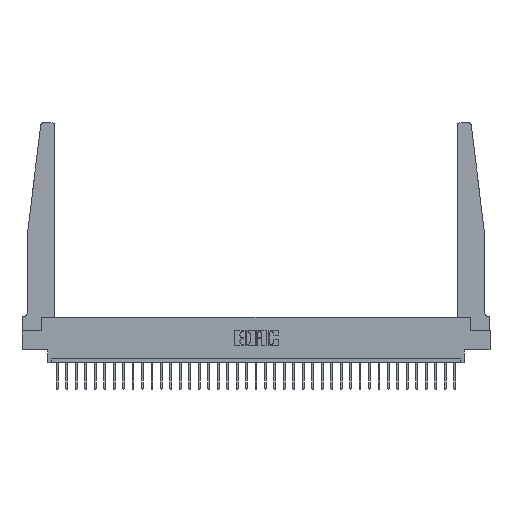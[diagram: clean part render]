
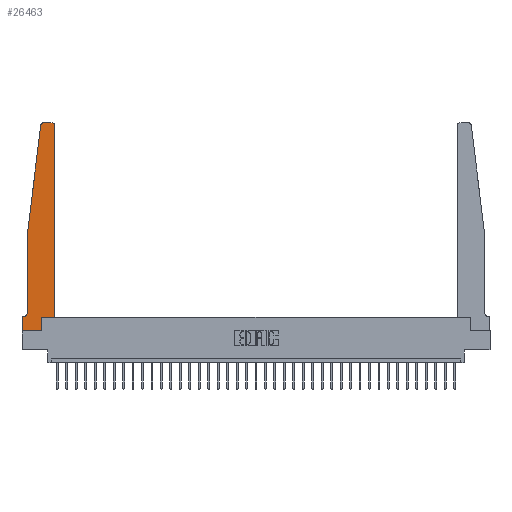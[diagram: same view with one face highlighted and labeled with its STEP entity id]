
A CAD part, top view. The second image highlights one B-rep face of the part: STEP entity #26463.
In plain terms, the highlighted planar face has unit normal (0, 0, 1).
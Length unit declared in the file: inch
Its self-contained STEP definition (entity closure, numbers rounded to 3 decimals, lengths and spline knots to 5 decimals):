
#137 = VERTEX_POINT ( 'NONE', #4157 ) ;
#386 = CARTESIAN_POINT ( 'NONE',  ( 0.27653, 2.72, 0.37 ) ) ;
#509 = VERTEX_POINT ( 'NONE', #14719 ) ;
#3121 = CARTESIAN_POINT ( 'NONE',  ( 0., 0., 0.37 ) ) ;
#3196 = DIRECTION ( 'NONE',  ( 0., -1., 0. ) ) ;
#3237 = LINE ( 'NONE', #26869, #28651 ) ;
#3584 = CARTESIAN_POINT ( 'NONE',  ( 0.425, 2.72, 0.37 ) ) ;
#4157 = CARTESIAN_POINT ( 'NONE',  ( 0.065, 0.2375, 0.37 ) ) ;
#4167 = LINE ( 'NONE', #28250, #23839 ) ;
#4971 = DIRECTION ( 'NONE',  ( 1., 0., 0. ) ) ;
#4999 = CIRCLE ( 'NONE', #12728, 0.03 ) ;
#5770 = CARTESIAN_POINT ( 'NONE',  ( 0., 0., 0.37 ) ) ;
#6089 = LINE ( 'NONE', #25825, #13481 ) ;
#6142 = DIRECTION ( 'NONE',  ( 0., 0., -1. ) ) ;
#6215 = DIRECTION ( 'NONE',  ( 1., 0., 0. ) ) ;
#7023 = VERTEX_POINT ( 'NONE', #16021 ) ;
#7190 = ORIENTED_EDGE ( 'NONE', *, *, #22446, .T. ) ;
#7372 = LINE ( 'NONE', #27103, #28190 ) ;
#8461 = CARTESIAN_POINT ( 'NONE',  ( 0., 0., 0.37 ) ) ;
#8720 = ORIENTED_EDGE ( 'NONE', *, *, #9805, .T. ) ;
#9675 = VECTOR ( 'NONE', #11392, 39.37008 ) ;
#9782 = ORIENTED_EDGE ( 'NONE', *, *, #12063, .T. ) ;
#9805 = EDGE_CURVE ( 'NONE', #7023, #137, #3237, .T. ) ;
#10181 = VERTEX_POINT ( 'NONE', #12892 ) ;
#10327 = EDGE_CURVE ( 'NONE', #31701, #31206, #7372, .T. ) ;
#10443 = CARTESIAN_POINT ( 'NONE',  ( 0.395, 2.72, 0.37 ) ) ;
#10842 = ORIENTED_EDGE ( 'NONE', *, *, #17889, .T. ) ;
#11392 = DIRECTION ( 'NONE',  ( -1., 0., 0. ) ) ;
#11553 = DIRECTION ( 'NONE',  ( 0., 0., 1. ) ) ;
#12063 = EDGE_CURVE ( 'NONE', #20946, #23874, #20159, .T. ) ;
#12728 = AXIS2_PLACEMENT_3D ( 'NONE', #386, #31696, #29286 ) ;
#12892 = CARTESIAN_POINT ( 'NONE',  ( 0.27653, 2.75, 0.37 ) ) ;
#12912 = CARTESIAN_POINT ( 'NONE',  ( 0.065, 1.25, 0.37 ) ) ;
#13356 = FACE_OUTER_BOUND ( 'NONE', #17643, .T. ) ;
#13382 = ORIENTED_EDGE ( 'NONE', *, *, #15493, .T. ) ;
#13399 = VERTEX_POINT ( 'NONE', #27915 ) ;
#13481 = VECTOR ( 'NONE', #28697, 39.37008 ) ;
#13879 = ORIENTED_EDGE ( 'NONE', *, *, #18957, .T. ) ;
#13944 = EDGE_CURVE ( 'NONE', #509, #20946, #23501, .T. ) ;
#14719 = CARTESIAN_POINT ( 'NONE',  ( 0.015, 0.1875, 0.37 ) ) ;
#15308 = DIRECTION ( 'NONE',  ( 1., 0., 0. ) ) ;
#15493 = EDGE_CURVE ( 'NONE', #13399, #10181, #17517, .T. ) ;
#15588 = CARTESIAN_POINT ( 'NONE',  ( 0.25, 2.75, 0.37 ) ) ;
#15610 = VECTOR ( 'NONE', #20330, 39.37008 ) ;
#15692 = CIRCLE ( 'NONE', #23404, 0.05 ) ;
#16021 = CARTESIAN_POINT ( 'NONE',  ( 0.065, 1.25, 0.37 ) ) ;
#17269 = CARTESIAN_POINT ( 'NONE',  ( 0.2605, 0.18, 0.37 ) ) ;
#17439 = ORIENTED_EDGE ( 'NONE', *, *, #10327, .T. ) ;
#17517 = LINE ( 'NONE', #15588, #28818 ) ;
#17643 = EDGE_LOOP ( 'NONE', ( #13382, #25815, #23143, #8720, #21719, #30098, #9782, #7190, #10842, #17439, #13879, #23720 ) ) ;
#17815 = AXIS2_PLACEMENT_3D ( 'NONE', #23206, #11553, #6215 ) ;
#17832 = DIRECTION ( 'NONE',  ( -1., 0., 0. ) ) ;
#17889 = EDGE_CURVE ( 'NONE', #25492, #31701, #6089, .T. ) ;
#18866 = EDGE_CURVE ( 'NONE', #26839, #7023, #25194, .T. ) ;
#18957 = EDGE_CURVE ( 'NONE', #31206, #28853, #4167, .T. ) ;
#19187 = CIRCLE ( 'NONE', #25423, 0.03 ) ;
#20159 = LINE ( 'NONE', #5770, #28754 ) ;
#20330 = DIRECTION ( 'NONE',  ( -0.122, -0.992, 0. ) ) ;
#20700 = CARTESIAN_POINT ( 'NONE',  ( 0.015, 0.2375, 0.37 ) ) ;
#20741 = EDGE_CURVE ( 'NONE', #28853, #13399, #19187, .T. ) ;
#20946 = VERTEX_POINT ( 'NONE', #31854 ) ;
#21719 = ORIENTED_EDGE ( 'NONE', *, *, #22892, .T. ) ;
#21734 = CARTESIAN_POINT ( 'NONE',  ( 0.425, 0.18, 0.37 ) ) ;
#22446 = EDGE_CURVE ( 'NONE', #23874, #25492, #23176, .T. ) ;
#22787 = DIRECTION ( 'NONE',  ( 0., -1., 0. ) ) ;
#22798 = CARTESIAN_POINT ( 'NONE',  ( 0.2605, 0., 0.37 ) ) ;
#22892 = EDGE_CURVE ( 'NONE', #137, #509, #15692, .T. ) ;
#23143 = ORIENTED_EDGE ( 'NONE', *, *, #18866, .T. ) ;
#23176 = LINE ( 'NONE', #8461, #24430 ) ;
#23206 = CARTESIAN_POINT ( 'NONE',  ( 0., 0.1875, 0.37 ) ) ;
#23404 = AXIS2_PLACEMENT_3D ( 'NONE', #20700, #6142, #28141 ) ;
#23501 = LINE ( 'NONE', #31212, #9675 ) ;
#23642 = DIRECTION ( 'NONE',  ( 1., 0., 0. ) ) ;
#23720 = ORIENTED_EDGE ( 'NONE', *, *, #20741, .T. ) ;
#23839 = VECTOR ( 'NONE', #24020, 39.37008 ) ;
#23874 = VERTEX_POINT ( 'NONE', #3121 ) ;
#24020 = DIRECTION ( 'NONE',  ( 0., 1., 0. ) ) ;
#24430 = VECTOR ( 'NONE', #23642, 39.37008 ) ;
#25194 = LINE ( 'NONE', #12912, #15610 ) ;
#25319 = DIRECTION ( 'NONE',  ( 0., 0., 1. ) ) ;
#25423 = AXIS2_PLACEMENT_3D ( 'NONE', #10443, #25319, #15308 ) ;
#25492 = VERTEX_POINT ( 'NONE', #22798 ) ;
#25815 = ORIENTED_EDGE ( 'NONE', *, *, #28330, .T. ) ;
#25825 = CARTESIAN_POINT ( 'NONE',  ( 0.2605, 0.18, 0.37 ) ) ;
#26463 = ADVANCED_FACE ( 'NONE', ( #13356 ), #30923, .T. ) ;
#26839 = VERTEX_POINT ( 'NONE', #29761 ) ;
#26869 = CARTESIAN_POINT ( 'NONE',  ( 0.065, 1.25, 0.37 ) ) ;
#27103 = CARTESIAN_POINT ( 'NONE',  ( 0.425, 0.18, 0.37 ) ) ;
#27915 = CARTESIAN_POINT ( 'NONE',  ( 0.395, 2.75, 0.37 ) ) ;
#28141 = DIRECTION ( 'NONE',  ( -1., 0., 0. ) ) ;
#28190 = VECTOR ( 'NONE', #4971, 39.37008 ) ;
#28250 = CARTESIAN_POINT ( 'NONE',  ( 0.425, 0.18, 0.37 ) ) ;
#28330 = EDGE_CURVE ( 'NONE', #10181, #26839, #4999, .T. ) ;
#28651 = VECTOR ( 'NONE', #22787, 39.37008 ) ;
#28697 = DIRECTION ( 'NONE',  ( 0., 1., 0. ) ) ;
#28754 = VECTOR ( 'NONE', #3196, 39.37008 ) ;
#28818 = VECTOR ( 'NONE', #17832, 39.37008 ) ;
#28853 = VERTEX_POINT ( 'NONE', #3584 ) ;
#29286 = DIRECTION ( 'NONE',  ( 1., 0., 0. ) ) ;
#29761 = CARTESIAN_POINT ( 'NONE',  ( 0.24675, 2.72367, 0.37 ) ) ;
#30098 = ORIENTED_EDGE ( 'NONE', *, *, #13944, .T. ) ;
#30923 = PLANE ( 'NONE',  #17815 ) ;
#31206 = VERTEX_POINT ( 'NONE', #21734 ) ;
#31212 = CARTESIAN_POINT ( 'NONE',  ( 0.065, 0.1875, 0.37 ) ) ;
#31696 = DIRECTION ( 'NONE',  ( 0., 0., 1. ) ) ;
#31701 = VERTEX_POINT ( 'NONE', #17269 ) ;
#31854 = CARTESIAN_POINT ( 'NONE',  ( 0., 0.1875, 0.37 ) ) ;
